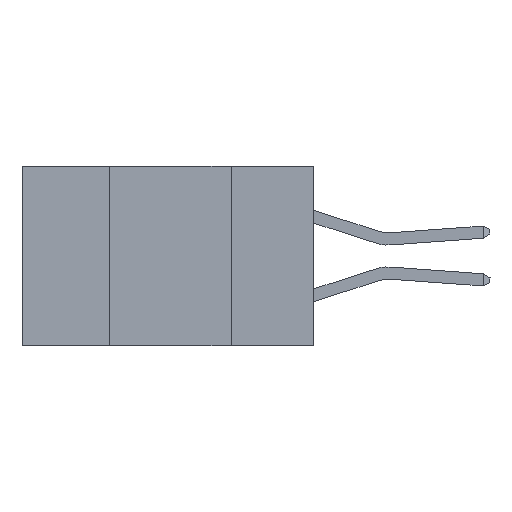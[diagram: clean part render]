
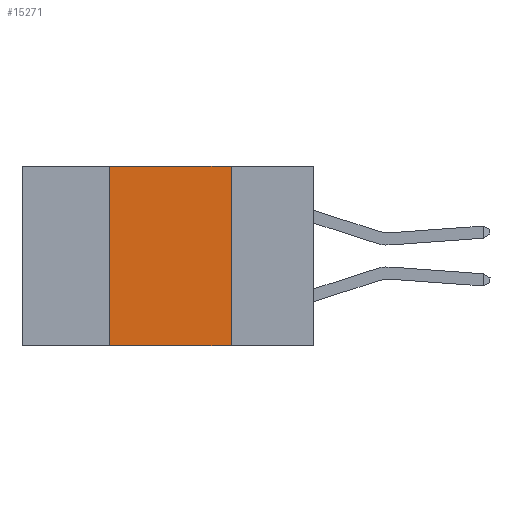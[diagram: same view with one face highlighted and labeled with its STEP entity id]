
A CAD part, left-side view. The second image highlights one B-rep face of the part: STEP entity #15271.
In plain terms, the highlighted planar face has unit normal (-1, 0, 0).
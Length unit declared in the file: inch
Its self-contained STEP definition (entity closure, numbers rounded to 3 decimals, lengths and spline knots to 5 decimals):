
#39 = ORIENTED_EDGE ( 'NONE', *, *, #16134, .F. ) ;
#163 = DIRECTION ( 'NONE',  ( 0., 0., -1. ) ) ;
#292 = ORIENTED_EDGE ( 'NONE', *, *, #9289, .F. ) ;
#522 = CARTESIAN_POINT ( 'NONE',  ( 0., 0.42, 0. ) ) ;
#857 = ORIENTED_EDGE ( 'NONE', *, *, #4635, .T. ) ;
#1071 = LINE ( 'NONE', #12925, #14982 ) ;
#1183 = VECTOR ( 'NONE', #9235, 39.37008 ) ;
#2865 = EDGE_LOOP ( 'NONE', ( #292, #12853, #39, #857 ) ) ;
#3624 = DIRECTION ( 'NONE',  ( 0., -1., 0. ) ) ;
#4342 = DIRECTION ( 'NONE',  ( 0., -1., 0. ) ) ;
#4635 = EDGE_CURVE ( 'NONE', #16679, #12002, #1071, .T. ) ;
#5556 = PLANE ( 'NONE',  #14232 ) ;
#5827 = VERTEX_POINT ( 'NONE', #522 ) ;
#6056 = VECTOR ( 'NONE', #4342, 39.37008 ) ;
#6922 = CARTESIAN_POINT ( 'NONE',  ( 0., 0.6, 0. ) ) ;
#7360 = CARTESIAN_POINT ( 'NONE',  ( 0., 0.17, 0. ) ) ;
#7607 = CARTESIAN_POINT ( 'NONE',  ( 0., 0.17, 0. ) ) ;
#7663 = DIRECTION ( 'NONE',  ( 0., 0., -1. ) ) ;
#8239 = DIRECTION ( 'NONE',  ( 1., 0., 0. ) ) ;
#8289 = CARTESIAN_POINT ( 'NONE',  ( 0., 0.42, -0.37 ) ) ;
#8558 = LINE ( 'NONE', #11423, #1183 ) ;
#9235 = DIRECTION ( 'NONE',  ( 0., 0., 1. ) ) ;
#9289 = EDGE_CURVE ( 'NONE', #9889, #12002, #16959, .T. ) ;
#9889 = VERTEX_POINT ( 'NONE', #7360 ) ;
#10094 = FACE_OUTER_BOUND ( 'NONE', #2865, .T. ) ;
#10276 = EDGE_CURVE ( 'NONE', #5827, #9889, #16815, .T. ) ;
#10878 = CARTESIAN_POINT ( 'NONE',  ( 0., 0.17, -0.37 ) ) ;
#11423 = CARTESIAN_POINT ( 'NONE',  ( 0., 0.42, 0. ) ) ;
#12002 = VERTEX_POINT ( 'NONE', #10878 ) ;
#12853 = ORIENTED_EDGE ( 'NONE', *, *, #10276, .F. ) ;
#12925 = CARTESIAN_POINT ( 'NONE',  ( 0., 0.6, -0.37 ) ) ;
#13365 = VECTOR ( 'NONE', #7663, 39.37008 ) ;
#14232 = AXIS2_PLACEMENT_3D ( 'NONE', #6922, #8239, #163 ) ;
#14914 = CARTESIAN_POINT ( 'NONE',  ( 0., 0.6, 0. ) ) ;
#14982 = VECTOR ( 'NONE', #3624, 39.37008 ) ;
#15271 = ADVANCED_FACE ( 'NONE', ( #10094 ), #5556, .F. ) ;
#16134 = EDGE_CURVE ( 'NONE', #16679, #5827, #8558, .T. ) ;
#16679 = VERTEX_POINT ( 'NONE', #8289 ) ;
#16815 = LINE ( 'NONE', #14914, #6056 ) ;
#16959 = LINE ( 'NONE', #7607, #13365 ) ;
